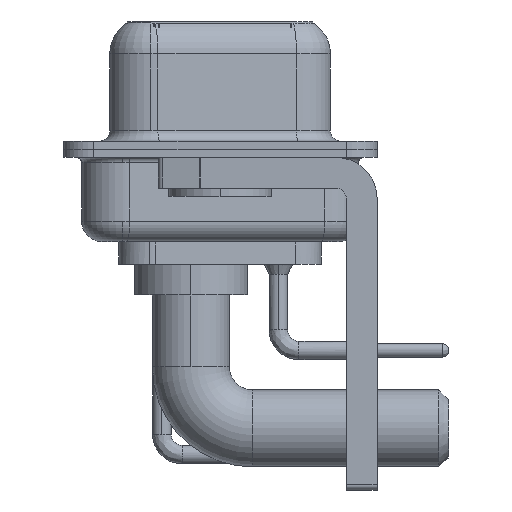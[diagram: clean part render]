
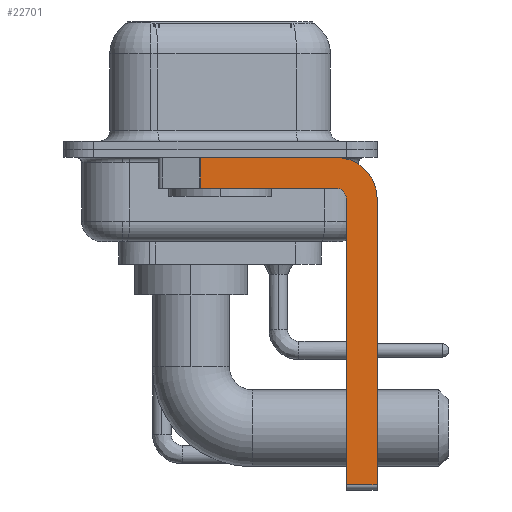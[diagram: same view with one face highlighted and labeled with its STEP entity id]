
A CAD part, left-side view. The second image highlights one B-rep face of the part: STEP entity #22701.
In plain terms, the highlighted planar face has unit normal (-1, 0, 0).
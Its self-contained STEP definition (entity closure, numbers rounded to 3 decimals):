
#186 = DIRECTION ( 'NONE',  ( 0., 0., -1. ) ) ;
#329 = CARTESIAN_POINT ( 'NONE',  ( -2.9, -6.15, -16.35 ) ) ;
#639 = CARTESIAN_POINT ( 'NONE',  ( -2.9, -5.65, -1.9 ) ) ;
#1479 = CARTESIAN_POINT ( 'NONE',  ( -2.9, -7.65, -2.4 ) ) ;
#2063 = CIRCLE ( 'NONE', #23478, 2. ) ;
#2371 = PLANE ( 'NONE',  #21704 ) ;
#2431 = CARTESIAN_POINT ( 'NONE',  ( -2.9, -6.15, -16.6 ) ) ;
#3064 = AXIS2_PLACEMENT_3D ( 'NONE', #3655, #29226, #27104 ) ;
#3655 = CARTESIAN_POINT ( 'NONE',  ( -2.9, -5.65, -2.4 ) ) ;
#3747 = DIRECTION ( 'NONE',  ( 0., -1., 0. ) ) ;
#3844 = ORIENTED_EDGE ( 'NONE', *, *, #8610, .T. ) ;
#4047 = CARTESIAN_POINT ( 'NONE',  ( -2.9, 3., -0.4 ) ) ;
#4390 = EDGE_CURVE ( 'NONE', #5688, #26393, #25617, .T. ) ;
#4420 = CARTESIAN_POINT ( 'NONE',  ( -2.9, -5.65, -0.4 ) ) ;
#4429 = VERTEX_POINT ( 'NONE', #639 ) ;
#4462 = CARTESIAN_POINT ( 'NONE',  ( -2.9, 0.978, -1.9 ) ) ;
#4756 = ORIENTED_EDGE ( 'NONE', *, *, #14343, .T. ) ;
#5150 = ORIENTED_EDGE ( 'NONE', *, *, #24890, .F. ) ;
#5688 = VERTEX_POINT ( 'NONE', #1479 ) ;
#6186 = CARTESIAN_POINT ( 'NONE',  ( -2.9, -5.65, -16.35 ) ) ;
#6920 = VERTEX_POINT ( 'NONE', #18525 ) ;
#7085 = DIRECTION ( 'NONE',  ( 0., 1., 0. ) ) ;
#8281 = VECTOR ( 'NONE', #27032, 1000. ) ;
#8469 = LINE ( 'NONE', #6186, #8281 ) ;
#8610 = EDGE_CURVE ( 'NONE', #20035, #26393, #8469, .T. ) ;
#8694 = EDGE_CURVE ( 'NONE', #4429, #14241, #9685, .T. ) ;
#9217 = LINE ( 'NONE', #4462, #10465 ) ;
#9616 = DIRECTION ( 'NONE',  ( 0., 0., 1. ) ) ;
#9685 = LINE ( 'NONE', #18959, #27229 ) ;
#10148 = CARTESIAN_POINT ( 'NONE',  ( -2.9, -6.15, -2.4 ) ) ;
#10198 = EDGE_LOOP ( 'NONE', ( #17079, #4756, #17442, #26164, #5150, #3844, #19944, #22492 ) ) ;
#10465 = VECTOR ( 'NONE', #11499, 1000. ) ;
#11252 = EDGE_CURVE ( 'NONE', #21868, #5688, #2063, .T. ) ;
#11356 = VERTEX_POINT ( 'NONE', #10148 ) ;
#11499 = DIRECTION ( 'NONE',  ( 0., 0., -1. ) ) ;
#11679 = DIRECTION ( 'NONE',  ( 1., 0., 0. ) ) ;
#11681 = CARTESIAN_POINT ( 'NONE',  ( -2.9, -5.65, -2.4 ) ) ;
#13025 = CARTESIAN_POINT ( 'NONE',  ( -2.9, 0.978, -1.9 ) ) ;
#14241 = VERTEX_POINT ( 'NONE', #13025 ) ;
#14343 = EDGE_CURVE ( 'NONE', #6920, #14241, #9217, .T. ) ;
#15939 = LINE ( 'NONE', #4047, #29368 ) ;
#17079 = ORIENTED_EDGE ( 'NONE', *, *, #19392, .F. ) ;
#17442 = ORIENTED_EDGE ( 'NONE', *, *, #8694, .F. ) ;
#17942 = VECTOR ( 'NONE', #186, 1000. ) ;
#18525 = CARTESIAN_POINT ( 'NONE',  ( -2.9, 0.978, -0.4 ) ) ;
#18660 = DIRECTION ( 'NONE',  ( 0., 0., -1. ) ) ;
#18959 = CARTESIAN_POINT ( 'NONE',  ( -2.9, -5.65, -1.9 ) ) ;
#19392 = EDGE_CURVE ( 'NONE', #6920, #21868, #15939, .T. ) ;
#19944 = ORIENTED_EDGE ( 'NONE', *, *, #4390, .F. ) ;
#20035 = VERTEX_POINT ( 'NONE', #329 ) ;
#20501 = DIRECTION ( 'NONE',  ( 1., 0., 0. ) ) ;
#20787 = VECTOR ( 'NONE', #9616, 1000. ) ;
#20956 = DIRECTION ( 'NONE',  ( 0., 0., -1. ) ) ;
#21704 = AXIS2_PLACEMENT_3D ( 'NONE', #11681, #20501, #20956 ) ;
#21868 = VERTEX_POINT ( 'NONE', #4420 ) ;
#22492 = ORIENTED_EDGE ( 'NONE', *, *, #11252, .F. ) ;
#22701 = ADVANCED_FACE ( 'NONE', ( #23221 ), #2371, .F. ) ;
#23218 = CARTESIAN_POINT ( 'NONE',  ( -2.9, -5.65, -2.4 ) ) ;
#23221 = FACE_OUTER_BOUND ( 'NONE', #10198, .T. ) ;
#23478 = AXIS2_PLACEMENT_3D ( 'NONE', #23218, #11679, #18660 ) ;
#23481 = CARTESIAN_POINT ( 'NONE',  ( -2.9, -7.65, -2.4 ) ) ;
#24084 = CARTESIAN_POINT ( 'NONE',  ( -2.9, -7.65, -16.35 ) ) ;
#24469 = CIRCLE ( 'NONE', #3064, 0.5 ) ;
#24890 = EDGE_CURVE ( 'NONE', #20035, #11356, #27724, .T. ) ;
#25617 = LINE ( 'NONE', #23481, #17942 ) ;
#26164 = ORIENTED_EDGE ( 'NONE', *, *, #27463, .F. ) ;
#26393 = VERTEX_POINT ( 'NONE', #24084 ) ;
#27032 = DIRECTION ( 'NONE',  ( 0., -1., 0. ) ) ;
#27104 = DIRECTION ( 'NONE',  ( 0., 0., 1. ) ) ;
#27229 = VECTOR ( 'NONE', #7085, 1000. ) ;
#27463 = EDGE_CURVE ( 'NONE', #11356, #4429, #24469, .T. ) ;
#27724 = LINE ( 'NONE', #2431, #20787 ) ;
#29226 = DIRECTION ( 'NONE',  ( -1., 0., 0. ) ) ;
#29368 = VECTOR ( 'NONE', #3747, 1000. ) ;
